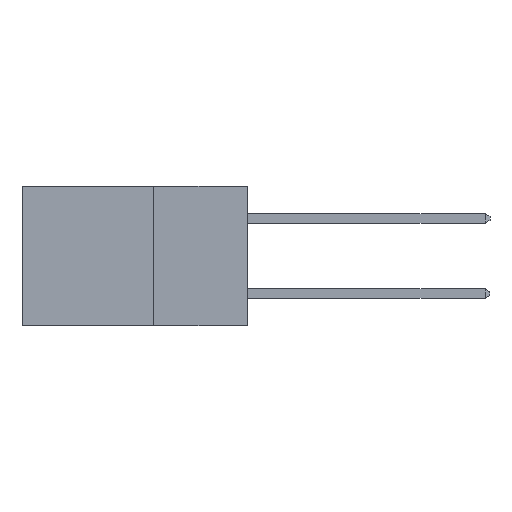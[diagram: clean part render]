
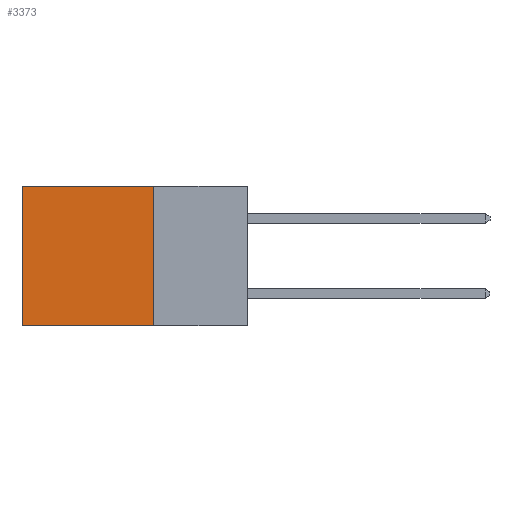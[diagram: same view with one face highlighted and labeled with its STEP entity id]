
A CAD part, left-side view. The second image highlights one B-rep face of the part: STEP entity #3373.
In plain terms, the highlighted planar face has unit normal (-1, 0, 0).
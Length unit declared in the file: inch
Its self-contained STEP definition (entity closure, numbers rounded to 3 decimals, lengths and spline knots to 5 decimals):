
#182 = CARTESIAN_POINT ( 'NONE',  ( 0.298, 0.25, 0. ) ) ;
#560 = DIRECTION ( 'NONE',  ( 0., 1., 0. ) ) ;
#594 = ORIENTED_EDGE ( 'NONE', *, *, #20255, .T. ) ;
#2628 = CARTESIAN_POINT ( 'NONE',  ( 0.298, 0.6, 0. ) ) ;
#3373 = ADVANCED_FACE ( 'NONE', ( #26443 ), #15269, .F. ) ;
#3674 = ORIENTED_EDGE ( 'NONE', *, *, #21230, .F. ) ;
#4426 = EDGE_CURVE ( 'NONE', #24005, #11011, #5990, .T. ) ;
#4612 = VECTOR ( 'NONE', #19327, 39.37008 ) ;
#5990 = LINE ( 'NONE', #182, #10919 ) ;
#6966 = EDGE_LOOP ( 'NONE', ( #594, #3674, #9733, #7927 ) ) ;
#7599 = DIRECTION ( 'NONE',  ( 0., 1., 0. ) ) ;
#7846 = VECTOR ( 'NONE', #7599, 39.37008 ) ;
#7927 = ORIENTED_EDGE ( 'NONE', *, *, #4426, .T. ) ;
#8128 = VERTEX_POINT ( 'NONE', #26689 ) ;
#9170 = EDGE_CURVE ( 'NONE', #24005, #20377, #12536, .T. ) ;
#9733 = ORIENTED_EDGE ( 'NONE', *, *, #9170, .F. ) ;
#10309 = AXIS2_PLACEMENT_3D ( 'NONE', #15292, #17654, #14753 ) ;
#10919 = VECTOR ( 'NONE', #560, 39.37008 ) ;
#11011 = VERTEX_POINT ( 'NONE', #22735 ) ;
#11819 = CARTESIAN_POINT ( 'NONE',  ( 0.298, 0.25, -0.37 ) ) ;
#12536 = LINE ( 'NONE', #23522, #17368 ) ;
#13248 = DIRECTION ( 'NONE',  ( 0., 0., -1. ) ) ;
#14076 = LINE ( 'NONE', #11819, #7846 ) ;
#14753 = DIRECTION ( 'NONE',  ( 0., 0., -1. ) ) ;
#15269 = PLANE ( 'NONE',  #10309 ) ;
#15292 = CARTESIAN_POINT ( 'NONE',  ( 0.298, 0.25, 0. ) ) ;
#17368 = VECTOR ( 'NONE', #13248, 39.37008 ) ;
#17654 = DIRECTION ( 'NONE',  ( 1., 0., 0. ) ) ;
#17675 = CARTESIAN_POINT ( 'NONE',  ( 0.298, 0.25, -0.37 ) ) ;
#19327 = DIRECTION ( 'NONE',  ( 0., 0., -1. ) ) ;
#20255 = EDGE_CURVE ( 'NONE', #11011, #8128, #26668, .T. ) ;
#20377 = VERTEX_POINT ( 'NONE', #17675 ) ;
#21230 = EDGE_CURVE ( 'NONE', #20377, #8128, #14076, .T. ) ;
#22735 = CARTESIAN_POINT ( 'NONE',  ( 0.298, 0.6, 0. ) ) ;
#23522 = CARTESIAN_POINT ( 'NONE',  ( 0.298, 0.25, 0. ) ) ;
#24005 = VERTEX_POINT ( 'NONE', #25415 ) ;
#25415 = CARTESIAN_POINT ( 'NONE',  ( 0.298, 0.25, 0. ) ) ;
#26443 = FACE_OUTER_BOUND ( 'NONE', #6966, .T. ) ;
#26668 = LINE ( 'NONE', #2628, #4612 ) ;
#26689 = CARTESIAN_POINT ( 'NONE',  ( 0.298, 0.6, -0.37 ) ) ;
